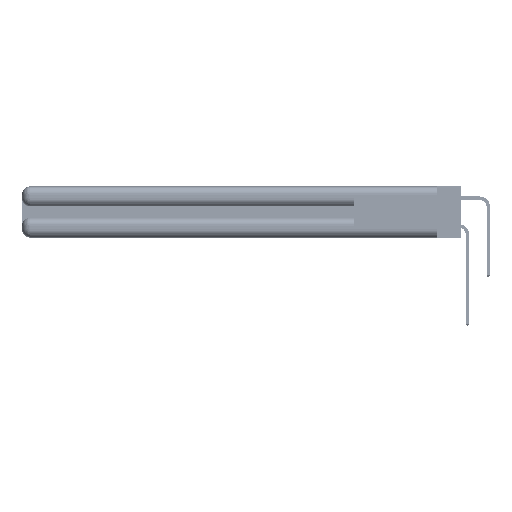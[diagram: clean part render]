
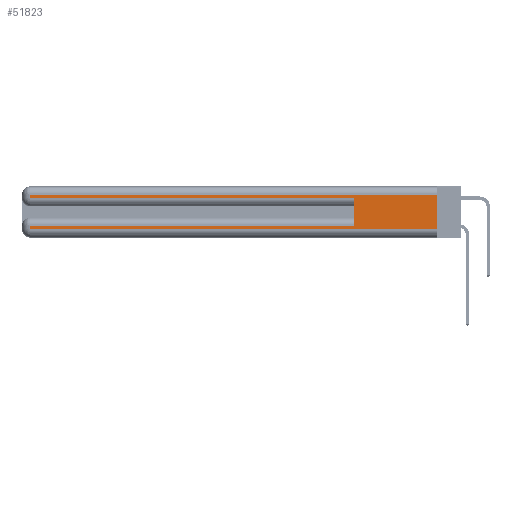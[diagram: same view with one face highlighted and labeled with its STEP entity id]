
A CAD part, left-side view. The second image highlights one B-rep face of the part: STEP entity #51823.
In plain terms, the highlighted planar face has unit normal (-1, 0, 0).
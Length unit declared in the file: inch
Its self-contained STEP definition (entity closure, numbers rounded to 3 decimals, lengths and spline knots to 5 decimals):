
#480 = EDGE_CURVE ( 'NONE', #50888, #52958, #27503, .T. ) ;
#585 = EDGE_LOOP ( 'NONE', ( #20722, #27618, #28511, #48134, #39048, #30699, #36683, #8061 ) ) ;
#1051 = EDGE_CURVE ( 'NONE', #48076, #50433, #43809, .T. ) ;
#1097 = VECTOR ( 'NONE', #26229, 39.37008 ) ;
#2530 = VECTOR ( 'NONE', #5254, 39.37008 ) ;
#3114 = AXIS2_PLACEMENT_3D ( 'NONE', #35665, #10575, #48285 ) ;
#5208 = VECTOR ( 'NONE', #16795, 39.37008 ) ;
#5254 = DIRECTION ( 'NONE',  ( 0., 1., 0. ) ) ;
#8061 = ORIENTED_EDGE ( 'NONE', *, *, #1051, .T. ) ;
#9706 = EDGE_CURVE ( 'NONE', #46824, #50433, #38560, .T. ) ;
#10575 = DIRECTION ( 'NONE',  ( 1., 0., 0. ) ) ;
#11410 = CARTESIAN_POINT ( 'NONE',  ( 0., 2.94, 0.285 ) ) ;
#12580 = CARTESIAN_POINT ( 'NONE',  ( 0., 0.6, 0.145 ) ) ;
#12757 = LINE ( 'NONE', #24283, #30496 ) ;
#15383 = DIRECTION ( 'NONE',  ( 0., 0., -1. ) ) ;
#16795 = DIRECTION ( 'NONE',  ( 0., 0., 1. ) ) ;
#17083 = EDGE_CURVE ( 'NONE', #53807, #52958, #12757, .T. ) ;
#17967 = CARTESIAN_POINT ( 'NONE',  ( 0., 0.6, 0.085 ) ) ;
#18360 = CARTESIAN_POINT ( 'NONE',  ( 0., 2.94, 0.06 ) ) ;
#18738 = CARTESIAN_POINT ( 'NONE',  ( 0., 2.94, 0.37 ) ) ;
#19555 = EDGE_CURVE ( 'NONE', #46824, #25950, #31487, .T. ) ;
#19567 = VECTOR ( 'NONE', #51568, 39.37008 ) ;
#20722 = ORIENTED_EDGE ( 'NONE', *, *, #9706, .F. ) ;
#21782 = EDGE_CURVE ( 'NONE', #25979, #48076, #46996, .T. ) ;
#24283 = CARTESIAN_POINT ( 'NONE',  ( 0., 0., 0.285 ) ) ;
#25950 = VERTEX_POINT ( 'NONE', #27616 ) ;
#25979 = VERTEX_POINT ( 'NONE', #39898 ) ;
#26229 = DIRECTION ( 'NONE',  ( 0., 0., -1. ) ) ;
#27424 = VECTOR ( 'NONE', #40781, 39.37008 ) ;
#27503 = LINE ( 'NONE', #12580, #5208 ) ;
#27616 = CARTESIAN_POINT ( 'NONE',  ( 0., 2.94, 0.31 ) ) ;
#27618 = ORIENTED_EDGE ( 'NONE', *, *, #19555, .T. ) ;
#28019 = CARTESIAN_POINT ( 'NONE',  ( 0., 0., 0.31 ) ) ;
#28511 = ORIENTED_EDGE ( 'NONE', *, *, #51215, .T. ) ;
#29978 = CARTESIAN_POINT ( 'NONE',  ( 0., 0., 0.06 ) ) ;
#30496 = VECTOR ( 'NONE', #53038, 39.37008 ) ;
#30699 = ORIENTED_EDGE ( 'NONE', *, *, #36874, .T. ) ;
#30838 = CARTESIAN_POINT ( 'NONE',  ( 0., 0., 0.06 ) ) ;
#31429 = PLANE ( 'NONE',  #3114 ) ;
#31487 = LINE ( 'NONE', #28019, #32813 ) ;
#32256 = DIRECTION ( 'NONE',  ( 0., 1., 0. ) ) ;
#32813 = VECTOR ( 'NONE', #32256, 39.37008 ) ;
#35665 = CARTESIAN_POINT ( 'NONE',  ( 0., 0., 0.37 ) ) ;
#36683 = ORIENTED_EDGE ( 'NONE', *, *, #21782, .T. ) ;
#36874 = EDGE_CURVE ( 'NONE', #50888, #25979, #37283, .T. ) ;
#37283 = LINE ( 'NONE', #42437, #2530 ) ;
#38560 = LINE ( 'NONE', #40596, #27424 ) ;
#39048 = ORIENTED_EDGE ( 'NONE', *, *, #480, .F. ) ;
#39692 = CARTESIAN_POINT ( 'NONE',  ( 0., 0., 0.31 ) ) ;
#39898 = CARTESIAN_POINT ( 'NONE',  ( 0., 2.94, 0.085 ) ) ;
#40596 = CARTESIAN_POINT ( 'NONE',  ( 0., 0., 0.37 ) ) ;
#40781 = DIRECTION ( 'NONE',  ( 0., 0., -1. ) ) ;
#42428 = VECTOR ( 'NONE', #15383, 39.37008 ) ;
#42437 = CARTESIAN_POINT ( 'NONE',  ( 0., 0., 0.085 ) ) ;
#43556 = CARTESIAN_POINT ( 'NONE',  ( 0., 0.6, 0.285 ) ) ;
#43809 = LINE ( 'NONE', #29978, #19567 ) ;
#44334 = FACE_OUTER_BOUND ( 'NONE', #585, .T. ) ;
#46824 = VERTEX_POINT ( 'NONE', #39692 ) ;
#46996 = LINE ( 'NONE', #18738, #1097 ) ;
#48076 = VERTEX_POINT ( 'NONE', #18360 ) ;
#48134 = ORIENTED_EDGE ( 'NONE', *, *, #17083, .T. ) ;
#48285 = DIRECTION ( 'NONE',  ( 0., 0., -1. ) ) ;
#49048 = CARTESIAN_POINT ( 'NONE',  ( 0., 2.94, 0.37 ) ) ;
#50433 = VERTEX_POINT ( 'NONE', #30838 ) ;
#50888 = VERTEX_POINT ( 'NONE', #17967 ) ;
#51215 = EDGE_CURVE ( 'NONE', #25950, #53807, #52929, .T. ) ;
#51568 = DIRECTION ( 'NONE',  ( 0., -1., 0. ) ) ;
#51823 = ADVANCED_FACE ( 'NONE', ( #44334 ), #31429, .F. ) ;
#52929 = LINE ( 'NONE', #49048, #42428 ) ;
#52958 = VERTEX_POINT ( 'NONE', #43556 ) ;
#53038 = DIRECTION ( 'NONE',  ( 0., -1., 0. ) ) ;
#53807 = VERTEX_POINT ( 'NONE', #11410 ) ;
